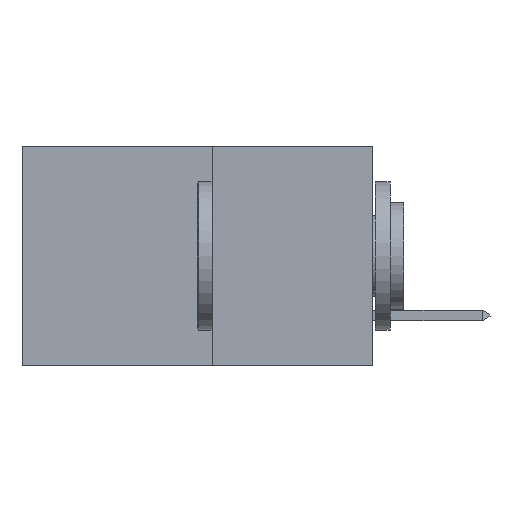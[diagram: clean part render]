
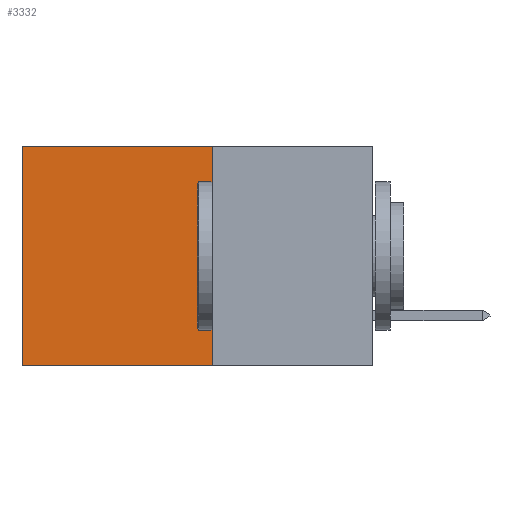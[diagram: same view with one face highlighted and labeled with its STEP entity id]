
A CAD part, left-side view. The second image highlights one B-rep face of the part: STEP entity #3332.
In plain terms, the highlighted planar face has unit normal (-1, 0, 0).
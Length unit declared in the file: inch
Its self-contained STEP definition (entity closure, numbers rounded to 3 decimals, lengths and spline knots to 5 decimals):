
#112 = CARTESIAN_POINT ( 'NONE',  ( 0.277, 0.59, -0.37 ) ) ;
#565 = VERTEX_POINT ( 'NONE', #7974 ) ;
#872 = CARTESIAN_POINT ( 'NONE',  ( 0.277, 0.27, -0.37 ) ) ;
#1673 = DIRECTION ( 'NONE',  ( 0., 1., 0. ) ) ;
#2248 = ORIENTED_EDGE ( 'NONE', *, *, #2717, .F. ) ;
#2717 = EDGE_CURVE ( 'NONE', #8777, #565, #5802, .T. ) ;
#3302 = EDGE_CURVE ( 'NONE', #8777, #5138, #5918, .T. ) ;
#3332 = ADVANCED_FACE ( 'NONE', ( #3568 ), #9111, .F. ) ;
#3568 = FACE_OUTER_BOUND ( 'NONE', #8527, .T. ) ;
#3707 = VECTOR ( 'NONE', #7844, 39.37008 ) ;
#3818 = VECTOR ( 'NONE', #9414, 39.37008 ) ;
#4195 = CARTESIAN_POINT ( 'NONE',  ( 0.277, 0.27, 0. ) ) ;
#4468 = LINE ( 'NONE', #112, #8699 ) ;
#4638 = AXIS2_PLACEMENT_3D ( 'NONE', #9176, #9073, #9067 ) ;
#4886 = VERTEX_POINT ( 'NONE', #9068 ) ;
#5138 = VERTEX_POINT ( 'NONE', #6973 ) ;
#5645 = DIRECTION ( 'NONE',  ( 0., 0., -1. ) ) ;
#5802 = LINE ( 'NONE', #8166, #3707 ) ;
#5918 = LINE ( 'NONE', #9360, #3818 ) ;
#6211 = ORIENTED_EDGE ( 'NONE', *, *, #9200, .F. ) ;
#6449 = LINE ( 'NONE', #872, #8094 ) ;
#6734 = ORIENTED_EDGE ( 'NONE', *, *, #3302, .T. ) ;
#6973 = CARTESIAN_POINT ( 'NONE',  ( 0.277, 0.59, 0. ) ) ;
#7844 = DIRECTION ( 'NONE',  ( 0., 0., -1. ) ) ;
#7974 = CARTESIAN_POINT ( 'NONE',  ( 0.277, 0.27, -0.37 ) ) ;
#8094 = VECTOR ( 'NONE', #1673, 39.37008 ) ;
#8118 = ORIENTED_EDGE ( 'NONE', *, *, #9663, .T. ) ;
#8166 = CARTESIAN_POINT ( 'NONE',  ( 0.277, 0.27, -0.37 ) ) ;
#8527 = EDGE_LOOP ( 'NONE', ( #8118, #6211, #2248, #6734 ) ) ;
#8699 = VECTOR ( 'NONE', #5645, 39.37008 ) ;
#8777 = VERTEX_POINT ( 'NONE', #4195 ) ;
#9067 = DIRECTION ( 'NONE',  ( 0., 0., -1. ) ) ;
#9068 = CARTESIAN_POINT ( 'NONE',  ( 0.277, 0.59, -0.37 ) ) ;
#9073 = DIRECTION ( 'NONE',  ( 1., 0., 0. ) ) ;
#9111 = PLANE ( 'NONE',  #4638 ) ;
#9176 = CARTESIAN_POINT ( 'NONE',  ( 0.277, 0.27, -0.37 ) ) ;
#9200 = EDGE_CURVE ( 'NONE', #565, #4886, #6449, .T. ) ;
#9360 = CARTESIAN_POINT ( 'NONE',  ( 0.277, 0.27, 0. ) ) ;
#9414 = DIRECTION ( 'NONE',  ( 0., 1., 0. ) ) ;
#9663 = EDGE_CURVE ( 'NONE', #5138, #4886, #4468, .T. ) ;
